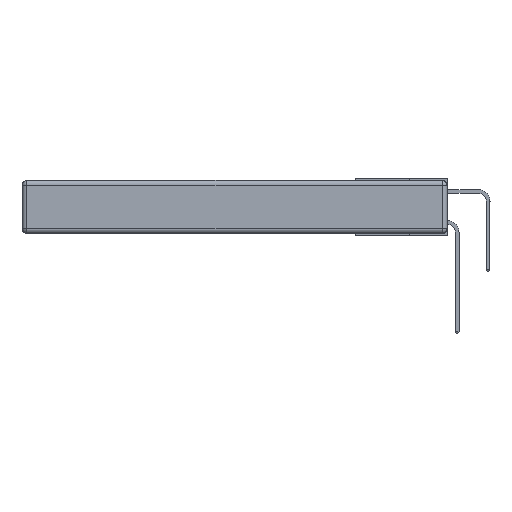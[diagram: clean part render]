
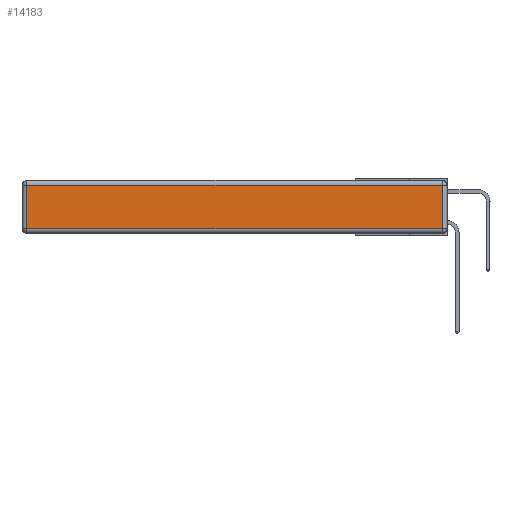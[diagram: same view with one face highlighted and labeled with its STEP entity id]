
A CAD part, left-side view. The second image highlights one B-rep face of the part: STEP entity #14183.
In plain terms, the highlighted planar face has unit normal (-1, 0, 0).
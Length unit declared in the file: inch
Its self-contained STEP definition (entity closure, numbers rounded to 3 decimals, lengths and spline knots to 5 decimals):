
#307 = CARTESIAN_POINT ( 'NONE',  ( 0., 2.72, -0.343 ) ) ;
#760 = DIRECTION ( 'NONE',  ( 0., -1., 0. ) ) ;
#1599 = LINE ( 'NONE', #7659, #12910 ) ;
#2262 = LINE ( 'NONE', #307, #14550 ) ;
#2268 = VERTEX_POINT ( 'NONE', #14898 ) ;
#2902 = LINE ( 'NONE', #15364, #18835 ) ;
#4480 = PLANE ( 'NONE',  #7667 ) ;
#4913 = VERTEX_POINT ( 'NONE', #6048 ) ;
#5080 = CARTESIAN_POINT ( 'NONE',  ( 0., 0.03, -0.343 ) ) ;
#6048 = CARTESIAN_POINT ( 'NONE',  ( 0., 2.72, -0.03 ) ) ;
#6430 = ORIENTED_EDGE ( 'NONE', *, *, #7367, .T. ) ;
#7211 = DIRECTION ( 'NONE',  ( 0., 0., 1. ) ) ;
#7367 = EDGE_CURVE ( 'NONE', #4913, #17107, #2262, .T. ) ;
#7659 = CARTESIAN_POINT ( 'NONE',  ( 0., 2.75, -0.03 ) ) ;
#7667 = AXIS2_PLACEMENT_3D ( 'NONE', #19289, #21370, #8758 ) ;
#8758 = DIRECTION ( 'NONE',  ( 0., 0., 1. ) ) ;
#8865 = EDGE_CURVE ( 'NONE', #17107, #16947, #2902, .T. ) ;
#8949 = DIRECTION ( 'NONE',  ( 0., 0., -1. ) ) ;
#9187 = EDGE_LOOP ( 'NONE', ( #24674, #12994, #9768, #6430 ) ) ;
#9768 = ORIENTED_EDGE ( 'NONE', *, *, #26740, .T. ) ;
#11347 = VECTOR ( 'NONE', #7211, 39.37008 ) ;
#11916 = FACE_OUTER_BOUND ( 'NONE', #9187, .T. ) ;
#12910 = VECTOR ( 'NONE', #16389, 39.37008 ) ;
#12994 = ORIENTED_EDGE ( 'NONE', *, *, #20909, .T. ) ;
#13244 = CARTESIAN_POINT ( 'NONE',  ( 0., 0.03, -0.313 ) ) ;
#14183 = ADVANCED_FACE ( 'NONE', ( #11916 ), #4480, .T. ) ;
#14550 = VECTOR ( 'NONE', #8949, 39.37008 ) ;
#14898 = CARTESIAN_POINT ( 'NONE',  ( 0., 0.03, -0.03 ) ) ;
#15364 = CARTESIAN_POINT ( 'NONE',  ( 0., 0., -0.313 ) ) ;
#16389 = DIRECTION ( 'NONE',  ( 0., 1., 0. ) ) ;
#16947 = VERTEX_POINT ( 'NONE', #13244 ) ;
#17107 = VERTEX_POINT ( 'NONE', #20506 ) ;
#18835 = VECTOR ( 'NONE', #760, 39.37008 ) ;
#19289 = CARTESIAN_POINT ( 'NONE',  ( 0., 0., -0.343 ) ) ;
#20506 = CARTESIAN_POINT ( 'NONE',  ( 0., 2.72, -0.313 ) ) ;
#20909 = EDGE_CURVE ( 'NONE', #16947, #2268, #22238, .T. ) ;
#21370 = DIRECTION ( 'NONE',  ( -1., 0., 0. ) ) ;
#22238 = LINE ( 'NONE', #5080, #11347 ) ;
#24674 = ORIENTED_EDGE ( 'NONE', *, *, #8865, .T. ) ;
#26740 = EDGE_CURVE ( 'NONE', #2268, #4913, #1599, .T. ) ;
